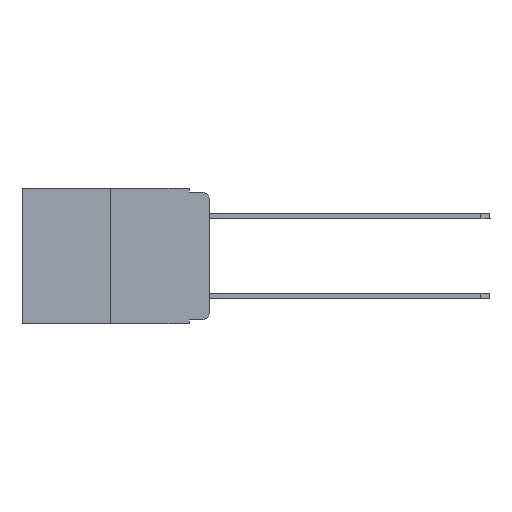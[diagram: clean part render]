
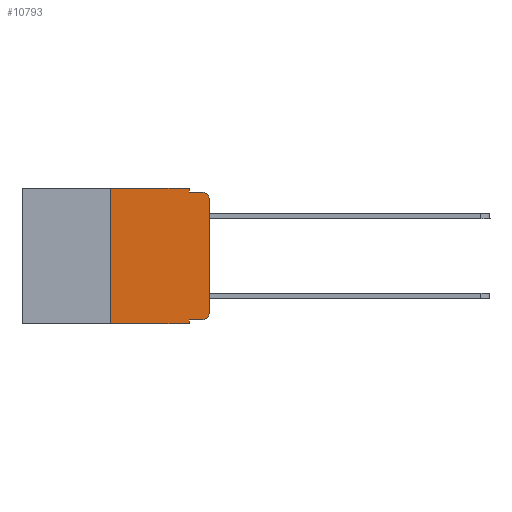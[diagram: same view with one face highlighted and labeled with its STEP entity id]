
A CAD part, left-side view. The second image highlights one B-rep face of the part: STEP entity #10793.
In plain terms, the highlighted planar face has unit normal (-1, 0, 0).
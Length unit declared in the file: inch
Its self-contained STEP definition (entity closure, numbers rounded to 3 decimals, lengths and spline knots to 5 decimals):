
#108 = DIRECTION ( 'NONE',  ( 1., 0., 0. ) ) ;
#153 = CARTESIAN_POINT ( 'NONE',  ( 0., 0., -0.313 ) ) ;
#164 = CIRCLE ( 'NONE', #2214, 0.02 ) ;
#368 = EDGE_CURVE ( 'NONE', #20779, #1235, #3721, .T. ) ;
#372 = ORIENTED_EDGE ( 'NONE', *, *, #12990, .T. ) ;
#1235 = VERTEX_POINT ( 'NONE', #15472 ) ;
#1274 = VECTOR ( 'NONE', #10975, 39.37008 ) ;
#1493 = ORIENTED_EDGE ( 'NONE', *, *, #2268, .T. ) ;
#1771 = LINE ( 'NONE', #17230, #1274 ) ;
#1862 = DIRECTION ( 'NONE',  ( 0., 0., -1. ) ) ;
#1872 = ORIENTED_EDGE ( 'NONE', *, *, #15641, .F. ) ;
#2054 = LINE ( 'NONE', #11894, #20756 ) ;
#2130 = CARTESIAN_POINT ( 'NONE',  ( 0., 0.473, 0. ) ) ;
#2194 = LINE ( 'NONE', #5083, #18344 ) ;
#2214 = AXIS2_PLACEMENT_3D ( 'NONE', #3535, #14915, #1862 ) ;
#2268 = EDGE_CURVE ( 'NONE', #7954, #17894, #2728, .T. ) ;
#2728 = LINE ( 'NONE', #7913, #14601 ) ;
#3132 = DIRECTION ( 'NONE',  ( 0., 0., -1. ) ) ;
#3229 = CARTESIAN_POINT ( 'NONE',  ( 0., 0.051, -0.343 ) ) ;
#3403 = VECTOR ( 'NONE', #10266, 39.37008 ) ;
#3535 = CARTESIAN_POINT ( 'NONE',  ( 0., 0.02, -0.313 ) ) ;
#3721 = CIRCLE ( 'NONE', #5267, 0.02 ) ;
#3999 = VECTOR ( 'NONE', #10428, 39.37008 ) ;
#4072 = VERTEX_POINT ( 'NONE', #11467 ) ;
#4341 = AXIS2_PLACEMENT_3D ( 'NONE', #11521, #108, #16426 ) ;
#5014 = LINE ( 'NONE', #14388, #16882 ) ;
#5083 = CARTESIAN_POINT ( 'NONE',  ( 0., 0.051, -0.01 ) ) ;
#5176 = CARTESIAN_POINT ( 'NONE',  ( 0., 0.051, -0.01 ) ) ;
#5267 = AXIS2_PLACEMENT_3D ( 'NONE', #9296, #6122, #9428 ) ;
#5508 = DIRECTION ( 'NONE',  ( 0., -1., 0. ) ) ;
#5614 = VERTEX_POINT ( 'NONE', #5176 ) ;
#6122 = DIRECTION ( 'NONE',  ( -1., 0., 0. ) ) ;
#6159 = ORIENTED_EDGE ( 'NONE', *, *, #11408, .T. ) ;
#6170 = ORIENTED_EDGE ( 'NONE', *, *, #7734, .F. ) ;
#6367 = ORIENTED_EDGE ( 'NONE', *, *, #15789, .F. ) ;
#6539 = DIRECTION ( 'NONE',  ( 0., -1., 0. ) ) ;
#7045 = DIRECTION ( 'NONE',  ( 0., 0., 1. ) ) ;
#7734 = EDGE_CURVE ( 'NONE', #7954, #10173, #1771, .T. ) ;
#7913 = CARTESIAN_POINT ( 'NONE',  ( 0., 0.473, -0.343 ) ) ;
#7954 = VERTEX_POINT ( 'NONE', #20386 ) ;
#8008 = LINE ( 'NONE', #19758, #3403 ) ;
#8820 = LINE ( 'NONE', #17029, #3999 ) ;
#8897 = EDGE_CURVE ( 'NONE', #10173, #14253, #10974, .T. ) ;
#9296 = CARTESIAN_POINT ( 'NONE',  ( 0., 0.02, -0.03 ) ) ;
#9428 = DIRECTION ( 'NONE',  ( 0., 0., -1. ) ) ;
#10173 = VERTEX_POINT ( 'NONE', #16380 ) ;
#10238 = EDGE_CURVE ( 'NONE', #16391, #20779, #2054, .T. ) ;
#10266 = DIRECTION ( 'NONE',  ( 0., 0., -1. ) ) ;
#10428 = DIRECTION ( 'NONE',  ( 0., -1., 0. ) ) ;
#10793 = ADVANCED_FACE ( 'NONE', ( #16895 ), #12993, .F. ) ;
#10974 = LINE ( 'NONE', #2130, #11708 ) ;
#10975 = DIRECTION ( 'NONE',  ( 0., 0., 1. ) ) ;
#11408 = EDGE_CURVE ( 'NONE', #18708, #4072, #8820, .T. ) ;
#11467 = CARTESIAN_POINT ( 'NONE',  ( 0., 0.02, -0.333 ) ) ;
#11521 = CARTESIAN_POINT ( 'NONE',  ( 0., 0.473, 0. ) ) ;
#11705 = CARTESIAN_POINT ( 'NONE',  ( 0., 0.051, 0. ) ) ;
#11708 = VECTOR ( 'NONE', #5508, 39.37008 ) ;
#11894 = CARTESIAN_POINT ( 'NONE',  ( 0., 0., 0. ) ) ;
#12990 = EDGE_CURVE ( 'NONE', #4072, #16391, #164, .T. ) ;
#12993 = PLANE ( 'NONE',  #4341 ) ;
#13465 = CARTESIAN_POINT ( 'NONE',  ( 0., 0., -0.03 ) ) ;
#14253 = VERTEX_POINT ( 'NONE', #11705 ) ;
#14388 = CARTESIAN_POINT ( 'NONE',  ( 0., 0.051, 0. ) ) ;
#14601 = VECTOR ( 'NONE', #19175, 39.37008 ) ;
#14915 = DIRECTION ( 'NONE',  ( -1., 0., 0. ) ) ;
#14926 = CARTESIAN_POINT ( 'NONE',  ( 0., 0.051, -0.333 ) ) ;
#15081 = ORIENTED_EDGE ( 'NONE', *, *, #19817, .F. ) ;
#15472 = CARTESIAN_POINT ( 'NONE',  ( 0., 0.02, -0.01 ) ) ;
#15641 = EDGE_CURVE ( 'NONE', #5614, #1235, #2194, .T. ) ;
#15789 = EDGE_CURVE ( 'NONE', #14253, #5614, #8008, .T. ) ;
#16380 = CARTESIAN_POINT ( 'NONE',  ( 0., 0.25, 0. ) ) ;
#16391 = VERTEX_POINT ( 'NONE', #153 ) ;
#16426 = DIRECTION ( 'NONE',  ( 0., 0., -1. ) ) ;
#16882 = VECTOR ( 'NONE', #3132, 39.37008 ) ;
#16895 = FACE_OUTER_BOUND ( 'NONE', #17790, .T. ) ;
#17029 = CARTESIAN_POINT ( 'NONE',  ( 0., 0.051, -0.333 ) ) ;
#17230 = CARTESIAN_POINT ( 'NONE',  ( 0., 0.25, 0. ) ) ;
#17790 = EDGE_LOOP ( 'NONE', ( #20025, #20477, #1872, #6367, #20312, #6170, #1493, #15081, #6159, #372 ) ) ;
#17894 = VERTEX_POINT ( 'NONE', #3229 ) ;
#18344 = VECTOR ( 'NONE', #6539, 39.37008 ) ;
#18708 = VERTEX_POINT ( 'NONE', #14926 ) ;
#19175 = DIRECTION ( 'NONE',  ( 0., -1., 0. ) ) ;
#19758 = CARTESIAN_POINT ( 'NONE',  ( 0., 0.051, 0. ) ) ;
#19817 = EDGE_CURVE ( 'NONE', #18708, #17894, #5014, .T. ) ;
#20025 = ORIENTED_EDGE ( 'NONE', *, *, #10238, .T. ) ;
#20312 = ORIENTED_EDGE ( 'NONE', *, *, #8897, .F. ) ;
#20386 = CARTESIAN_POINT ( 'NONE',  ( 0., 0.25, -0.343 ) ) ;
#20477 = ORIENTED_EDGE ( 'NONE', *, *, #368, .T. ) ;
#20756 = VECTOR ( 'NONE', #7045, 39.37008 ) ;
#20779 = VERTEX_POINT ( 'NONE', #13465 ) ;
